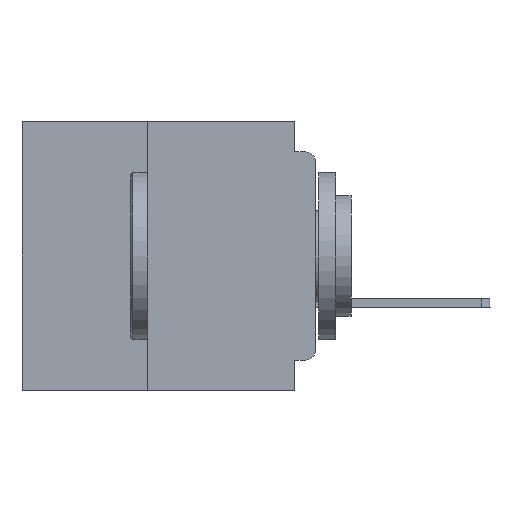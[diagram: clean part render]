
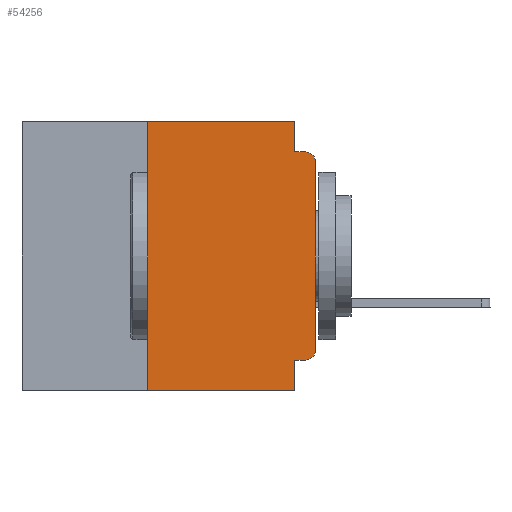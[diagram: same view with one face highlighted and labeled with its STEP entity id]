
A CAD part, left-side view. The second image highlights one B-rep face of the part: STEP entity #54256.
In plain terms, the highlighted planar face has unit normal (-1, 0, 0).
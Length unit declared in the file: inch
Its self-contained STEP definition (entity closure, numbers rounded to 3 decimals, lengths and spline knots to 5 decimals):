
#741 = DIRECTION ( 'NONE',  ( 0., -1., 0. ) ) ;
#795 = CARTESIAN_POINT ( 'NONE',  ( 0., 0.031, -0.045 ) ) ;
#913 = EDGE_CURVE ( 'NONE', #10618, #17953, #5515, .T. ) ;
#1140 = EDGE_CURVE ( 'NONE', #12972, #24564, #56586, .T. ) ;
#1813 = AXIS2_PLACEMENT_3D ( 'NONE', #65949, #35112, #3815 ) ;
#2020 = DIRECTION ( 'NONE',  ( 1., 0., 0. ) ) ;
#2169 = CARTESIAN_POINT ( 'NONE',  ( 0., 0., -0.34 ) ) ;
#2985 = VECTOR ( 'NONE', #741, 39.37008 ) ;
#3815 = DIRECTION ( 'NONE',  ( 0., 0., -1. ) ) ;
#3979 = DIRECTION ( 'NONE',  ( -1., 0., 0. ) ) ;
#4907 = CARTESIAN_POINT ( 'NONE',  ( 0., 0.031, -0.4 ) ) ;
#5515 = CIRCLE ( 'NONE', #22989, 0.015 ) ;
#6511 = DIRECTION ( 'NONE',  ( 0., -1., 0. ) ) ;
#7323 = CARTESIAN_POINT ( 'NONE',  ( 0., 0.031, 0. ) ) ;
#7370 = EDGE_CURVE ( 'NONE', #20268, #12972, #9753, .T. ) ;
#7749 = CARTESIAN_POINT ( 'NONE',  ( 0., 0.031, -0.4 ) ) ;
#9677 = VERTEX_POINT ( 'NONE', #795 ) ;
#9753 = LINE ( 'NONE', #46188, #63197 ) ;
#9870 = ORIENTED_EDGE ( 'NONE', *, *, #28393, .F. ) ;
#10618 = VERTEX_POINT ( 'NONE', #40320 ) ;
#10950 = ORIENTED_EDGE ( 'NONE', *, *, #40258, .F. ) ;
#12344 = DIRECTION ( 'NONE',  ( 0., -1., 0. ) ) ;
#12387 = CARTESIAN_POINT ( 'NONE',  ( 0., 0.437, 0. ) ) ;
#12740 = ORIENTED_EDGE ( 'NONE', *, *, #22712, .F. ) ;
#12972 = VERTEX_POINT ( 'NONE', #30049 ) ;
#13263 = VECTOR ( 'NONE', #54013, 39.37008 ) ;
#14226 = CARTESIAN_POINT ( 'NONE',  ( 0., 0.031, -0.355 ) ) ;
#14975 = DIRECTION ( 'NONE',  ( 0., 0., 1. ) ) ;
#15274 = DIRECTION ( 'NONE',  ( 0., 0., -1. ) ) ;
#16958 = VERTEX_POINT ( 'NONE', #61563 ) ;
#17953 = VERTEX_POINT ( 'NONE', #2169 ) ;
#18742 = CARTESIAN_POINT ( 'NONE',  ( 0., 0., -0.355 ) ) ;
#19724 = LINE ( 'NONE', #4907, #59273 ) ;
#20268 = VERTEX_POINT ( 'NONE', #63099 ) ;
#20695 = DIRECTION ( 'NONE',  ( 0., 0., 1. ) ) ;
#21392 = LINE ( 'NONE', #18742, #60973 ) ;
#22712 = EDGE_CURVE ( 'NONE', #61528, #40348, #19724, .T. ) ;
#22915 = PLANE ( 'NONE',  #43365 ) ;
#22989 = AXIS2_PLACEMENT_3D ( 'NONE', #35275, #3979, #40418 ) ;
#23364 = ORIENTED_EDGE ( 'NONE', *, *, #53123, .T. ) ;
#24444 = CARTESIAN_POINT ( 'NONE',  ( 0., 0., -0.06 ) ) ;
#24564 = VERTEX_POINT ( 'NONE', #30969 ) ;
#25743 = CARTESIAN_POINT ( 'NONE',  ( 0., 0., 0. ) ) ;
#28135 = CIRCLE ( 'NONE', #1813, 0.015 ) ;
#28393 = EDGE_CURVE ( 'NONE', #24564, #9677, #54514, .T. ) ;
#30049 = CARTESIAN_POINT ( 'NONE',  ( 0., 0.25, 0. ) ) ;
#30969 = CARTESIAN_POINT ( 'NONE',  ( 0., 0.031, 0. ) ) ;
#32530 = CARTESIAN_POINT ( 'NONE',  ( 0., 0.437, -0.4 ) ) ;
#34041 = ORIENTED_EDGE ( 'NONE', *, *, #1140, .F. ) ;
#34443 = VECTOR ( 'NONE', #12344, 39.37008 ) ;
#34658 = EDGE_CURVE ( 'NONE', #10618, #61528, #21392, .T. ) ;
#35112 = DIRECTION ( 'NONE',  ( -1., 0., 0. ) ) ;
#35275 = CARTESIAN_POINT ( 'NONE',  ( 0., 0.015, -0.34 ) ) ;
#35545 = EDGE_CURVE ( 'NONE', #17953, #49911, #55960, .T. ) ;
#36080 = FACE_OUTER_BOUND ( 'NONE', #52165, .T. ) ;
#36692 = VECTOR ( 'NONE', #6511, 39.37008 ) ;
#38528 = DIRECTION ( 'NONE',  ( 0., 0., -1. ) ) ;
#40258 = EDGE_CURVE ( 'NONE', #9677, #16958, #48046, .T. ) ;
#40320 = CARTESIAN_POINT ( 'NONE',  ( 0., 0.015, -0.355 ) ) ;
#40348 = VERTEX_POINT ( 'NONE', #7749 ) ;
#40418 = DIRECTION ( 'NONE',  ( 0., 0., -1. ) ) ;
#41686 = ORIENTED_EDGE ( 'NONE', *, *, #35545, .T. ) ;
#42258 = VECTOR ( 'NONE', #20695, 39.37008 ) ;
#43365 = AXIS2_PLACEMENT_3D ( 'NONE', #12387, #2020, #38528 ) ;
#43375 = CARTESIAN_POINT ( 'NONE',  ( 0., 0., -0.045 ) ) ;
#43452 = EDGE_CURVE ( 'NONE', #20268, #40348, #51929, .T. ) ;
#46188 = CARTESIAN_POINT ( 'NONE',  ( 0., 0.25, -0.4 ) ) ;
#48046 = LINE ( 'NONE', #43375, #34443 ) ;
#48057 = ORIENTED_EDGE ( 'NONE', *, *, #34658, .F. ) ;
#49669 = DIRECTION ( 'NONE',  ( 0., 1., 0. ) ) ;
#49911 = VERTEX_POINT ( 'NONE', #24444 ) ;
#51081 = ORIENTED_EDGE ( 'NONE', *, *, #43452, .T. ) ;
#51929 = LINE ( 'NONE', #32530, #36692 ) ;
#52165 = EDGE_LOOP ( 'NONE', ( #41686, #23364, #10950, #9870, #34041, #64299, #51081, #12740, #48057, #52794 ) ) ;
#52794 = ORIENTED_EDGE ( 'NONE', *, *, #913, .T. ) ;
#53123 = EDGE_CURVE ( 'NONE', #49911, #16958, #28135, .T. ) ;
#54013 = DIRECTION ( 'NONE',  ( 0., 0., -1. ) ) ;
#54256 = ADVANCED_FACE ( 'NONE', ( #36080 ), #22915, .F. ) ;
#54514 = LINE ( 'NONE', #7323, #13263 ) ;
#55960 = LINE ( 'NONE', #25743, #42258 ) ;
#56586 = LINE ( 'NONE', #57699, #2985 ) ;
#57699 = CARTESIAN_POINT ( 'NONE',  ( 0., 0.437, 0. ) ) ;
#59273 = VECTOR ( 'NONE', #15274, 39.37008 ) ;
#60973 = VECTOR ( 'NONE', #49669, 39.37008 ) ;
#61528 = VERTEX_POINT ( 'NONE', #14226 ) ;
#61563 = CARTESIAN_POINT ( 'NONE',  ( 0., 0.015, -0.045 ) ) ;
#63099 = CARTESIAN_POINT ( 'NONE',  ( 0., 0.25, -0.4 ) ) ;
#63197 = VECTOR ( 'NONE', #14975, 39.37008 ) ;
#64299 = ORIENTED_EDGE ( 'NONE', *, *, #7370, .F. ) ;
#65949 = CARTESIAN_POINT ( 'NONE',  ( 0., 0.015, -0.06 ) ) ;
